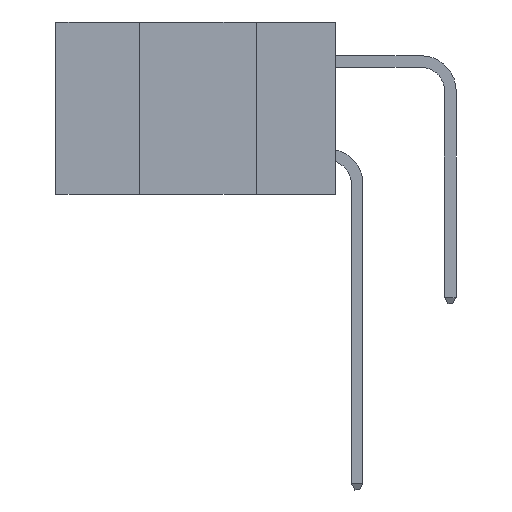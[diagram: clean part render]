
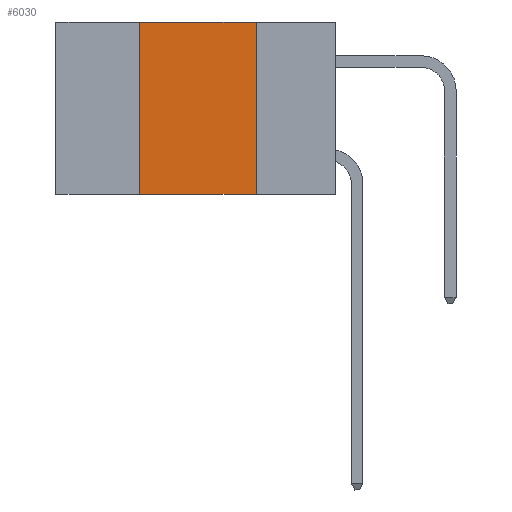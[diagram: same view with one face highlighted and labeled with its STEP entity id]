
A CAD part, left-side view. The second image highlights one B-rep face of the part: STEP entity #6030.
In plain terms, the highlighted planar face has unit normal (-1, 0, 0).
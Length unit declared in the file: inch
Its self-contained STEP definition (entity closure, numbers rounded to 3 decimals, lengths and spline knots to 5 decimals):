
#1172 = FACE_OUTER_BOUND ( 'NONE', #4547, .T. ) ;
#1575 = EDGE_CURVE ( 'NONE', #4090, #6902, #9633, .T. ) ;
#1804 = DIRECTION ( 'NONE',  ( 1., 0., 0. ) ) ;
#4090 = VERTEX_POINT ( 'NONE', #10756 ) ;
#4356 = ORIENTED_EDGE ( 'NONE', *, *, #9479, .F. ) ;
#4540 = CARTESIAN_POINT ( 'NONE',  ( 0., 0.6, 0. ) ) ;
#4547 = EDGE_LOOP ( 'NONE', ( #4356, #9773, #4675, #10103 ) ) ;
#4675 = ORIENTED_EDGE ( 'NONE', *, *, #10100, .F. ) ;
#4800 = EDGE_CURVE ( 'NONE', #11984, #9500, #10046, .T. ) ;
#5658 = LINE ( 'NONE', #12912, #11132 ) ;
#5795 = PLANE ( 'NONE',  #9095 ) ;
#6030 = ADVANCED_FACE ( 'NONE', ( #1172 ), #5795, .F. ) ;
#6133 = CARTESIAN_POINT ( 'NONE',  ( 0., 0.17, 0. ) ) ;
#6430 = VECTOR ( 'NONE', #9869, 39.37008 ) ;
#6506 = DIRECTION ( 'NONE',  ( 0., -1., 0. ) ) ;
#6815 = DIRECTION ( 'NONE',  ( 0., 0., -1. ) ) ;
#6902 = VERTEX_POINT ( 'NONE', #6133 ) ;
#7722 = LINE ( 'NONE', #8831, #6430 ) ;
#7989 = CARTESIAN_POINT ( 'NONE',  ( 0., 0.42, -0.37 ) ) ;
#8831 = CARTESIAN_POINT ( 'NONE',  ( 0., 0.42, 0. ) ) ;
#8895 = DIRECTION ( 'NONE',  ( 0., 0., -1. ) ) ;
#9095 = AXIS2_PLACEMENT_3D ( 'NONE', #11923, #1804, #8895 ) ;
#9479 = EDGE_CURVE ( 'NONE', #6902, #9500, #5658, .T. ) ;
#9500 = VERTEX_POINT ( 'NONE', #10947 ) ;
#9633 = LINE ( 'NONE', #4540, #9944 ) ;
#9773 = ORIENTED_EDGE ( 'NONE', *, *, #1575, .F. ) ;
#9869 = DIRECTION ( 'NONE',  ( 0., 0., 1. ) ) ;
#9944 = VECTOR ( 'NONE', #6506, 39.37008 ) ;
#10005 = CARTESIAN_POINT ( 'NONE',  ( 0., 0.6, -0.37 ) ) ;
#10046 = LINE ( 'NONE', #10005, #12415 ) ;
#10100 = EDGE_CURVE ( 'NONE', #11984, #4090, #7722, .T. ) ;
#10103 = ORIENTED_EDGE ( 'NONE', *, *, #4800, .T. ) ;
#10756 = CARTESIAN_POINT ( 'NONE',  ( 0., 0.42, 0. ) ) ;
#10947 = CARTESIAN_POINT ( 'NONE',  ( 0., 0.17, -0.37 ) ) ;
#11132 = VECTOR ( 'NONE', #6815, 39.37008 ) ;
#11923 = CARTESIAN_POINT ( 'NONE',  ( 0., 0.6, 0. ) ) ;
#11984 = VERTEX_POINT ( 'NONE', #7989 ) ;
#12038 = DIRECTION ( 'NONE',  ( 0., -1., 0. ) ) ;
#12415 = VECTOR ( 'NONE', #12038, 39.37008 ) ;
#12912 = CARTESIAN_POINT ( 'NONE',  ( 0., 0.17, 0. ) ) ;
